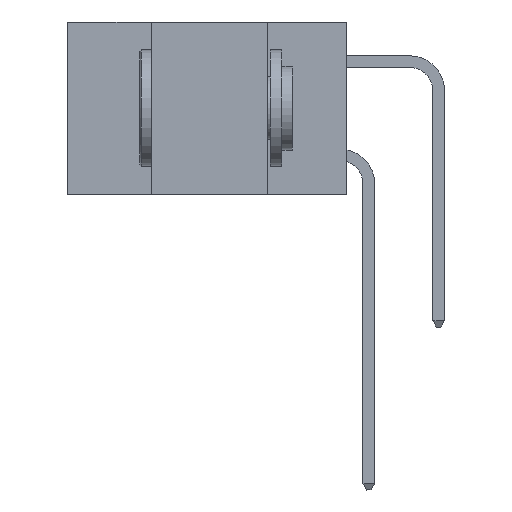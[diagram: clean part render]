
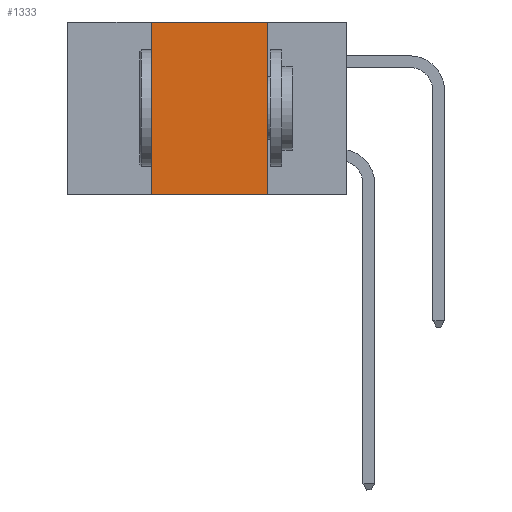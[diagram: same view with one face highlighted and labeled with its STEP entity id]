
A CAD part, left-side view. The second image highlights one B-rep face of the part: STEP entity #1333.
In plain terms, the highlighted planar face has unit normal (-1, 0, 0).
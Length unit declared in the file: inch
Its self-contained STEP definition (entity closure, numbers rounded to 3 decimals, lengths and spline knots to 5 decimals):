
#959 = VECTOR ( 'NONE', #10146, 39.37008 ) ;
#1333 = ADVANCED_FACE ( 'NONE', ( #12412 ), #12532, .F. ) ;
#2806 = ORIENTED_EDGE ( 'NONE', *, *, #26871, .F. ) ;
#3592 = DIRECTION ( 'NONE',  ( 0., -1., 0. ) ) ;
#4135 = LINE ( 'NONE', #6980, #17146 ) ;
#4725 = VERTEX_POINT ( 'NONE', #17542 ) ;
#5277 = ORIENTED_EDGE ( 'NONE', *, *, #13159, .T. ) ;
#6980 = CARTESIAN_POINT ( 'NONE',  ( 0., 0.42, 0. ) ) ;
#7486 = CARTESIAN_POINT ( 'NONE',  ( 0., 0.17, -0.37 ) ) ;
#10146 = DIRECTION ( 'NONE',  ( 0., -1., 0. ) ) ;
#10276 = CARTESIAN_POINT ( 'NONE',  ( 0., 0.42, -0.37 ) ) ;
#11598 = CARTESIAN_POINT ( 'NONE',  ( 0., 0.17, 0. ) ) ;
#11960 = DIRECTION ( 'NONE',  ( 0., 0., -1. ) ) ;
#12068 = DIRECTION ( 'NONE',  ( 1., 0., 0. ) ) ;
#12219 = CARTESIAN_POINT ( 'NONE',  ( 0., 0.6, 0. ) ) ;
#12412 = FACE_OUTER_BOUND ( 'NONE', #33077, .T. ) ;
#12532 = PLANE ( 'NONE',  #18616 ) ;
#12845 = EDGE_CURVE ( 'NONE', #4725, #26171, #21691, .T. ) ;
#13159 = EDGE_CURVE ( 'NONE', #18613, #20519, #18525, .T. ) ;
#16655 = ORIENTED_EDGE ( 'NONE', *, *, #12845, .F. ) ;
#17146 = VECTOR ( 'NONE', #17395, 39.37008 ) ;
#17395 = DIRECTION ( 'NONE',  ( 0., 0., 1. ) ) ;
#17542 = CARTESIAN_POINT ( 'NONE',  ( 0., 0.42, 0. ) ) ;
#18525 = LINE ( 'NONE', #21697, #19334 ) ;
#18613 = VERTEX_POINT ( 'NONE', #10276 ) ;
#18616 = AXIS2_PLACEMENT_3D ( 'NONE', #12219, #12068, #11960 ) ;
#19334 = VECTOR ( 'NONE', #3592, 39.37008 ) ;
#20519 = VERTEX_POINT ( 'NONE', #7486 ) ;
#21691 = LINE ( 'NONE', #25505, #959 ) ;
#21697 = CARTESIAN_POINT ( 'NONE',  ( 0., 0.6, -0.37 ) ) ;
#21743 = EDGE_CURVE ( 'NONE', #18613, #4725, #4135, .T. ) ;
#24338 = DIRECTION ( 'NONE',  ( 0., 0., -1. ) ) ;
#25037 = ORIENTED_EDGE ( 'NONE', *, *, #21743, .F. ) ;
#25505 = CARTESIAN_POINT ( 'NONE',  ( 0., 0.6, 0. ) ) ;
#25612 = LINE ( 'NONE', #11598, #32409 ) ;
#26171 = VERTEX_POINT ( 'NONE', #29198 ) ;
#26871 = EDGE_CURVE ( 'NONE', #26171, #20519, #25612, .T. ) ;
#29198 = CARTESIAN_POINT ( 'NONE',  ( 0., 0.17, 0. ) ) ;
#32409 = VECTOR ( 'NONE', #24338, 39.37008 ) ;
#33077 = EDGE_LOOP ( 'NONE', ( #2806, #16655, #25037, #5277 ) ) ;
